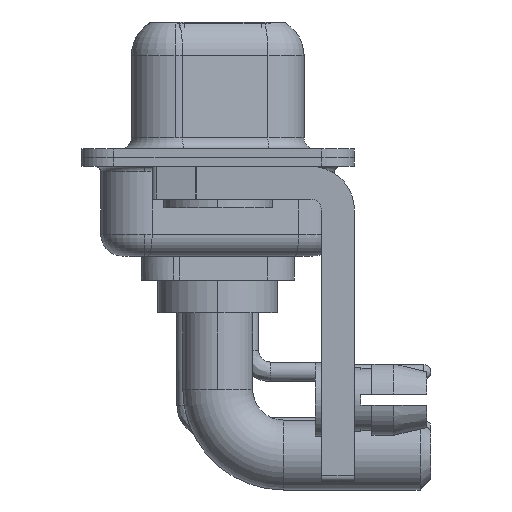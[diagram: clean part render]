
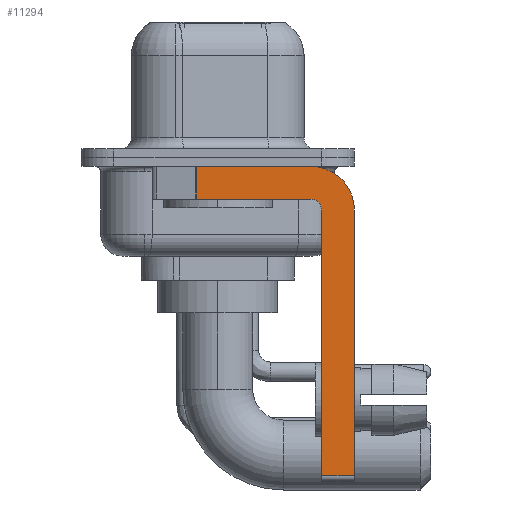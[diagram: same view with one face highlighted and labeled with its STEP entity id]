
A CAD part, left-side view. The second image highlights one B-rep face of the part: STEP entity #11294.
In plain terms, the highlighted planar face has unit normal (-1, 0, 0).
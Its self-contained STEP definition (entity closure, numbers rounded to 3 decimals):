
#166 = VERTEX_POINT ( 'NONE', #17908 ) ;
#473 = VERTEX_POINT ( 'NONE', #15379 ) ;
#1239 = ORIENTED_EDGE ( 'NONE', *, *, #25245, .F. ) ;
#1718 = VECTOR ( 'NONE', #11617, 1000. ) ;
#2003 = CARTESIAN_POINT ( 'NONE',  ( -2.9, -6.25, -2.4 ) ) ;
#2008 = VECTOR ( 'NONE', #10098, 1000. ) ;
#2915 = ORIENTED_EDGE ( 'NONE', *, *, #24611, .F. ) ;
#3667 = PLANE ( 'NONE',  #7235 ) ;
#5119 = CARTESIAN_POINT ( 'NONE',  ( -2.9, 0.978, -1.9 ) ) ;
#5285 = EDGE_CURVE ( 'NONE', #21362, #473, #16288, .T. ) ;
#5353 = CIRCLE ( 'NONE', #13408, 0.5 ) ;
#6689 = CARTESIAN_POINT ( 'NONE',  ( -2.9, -4.25, -2.4 ) ) ;
#6922 = VECTOR ( 'NONE', #20558, 1000. ) ;
#7119 = CARTESIAN_POINT ( 'NONE',  ( -2.9, -4.25, -1.9 ) ) ;
#7217 = VERTEX_POINT ( 'NONE', #15669 ) ;
#7235 = AXIS2_PLACEMENT_3D ( 'NONE', #11904, #17581, #11758 ) ;
#9989 = CARTESIAN_POINT ( 'NONE',  ( -2.9, -4.25, -0.4 ) ) ;
#10098 = DIRECTION ( 'NONE',  ( 0., 0., -1. ) ) ;
#11145 = DIRECTION ( 'NONE',  ( 0., -1., 0. ) ) ;
#11294 = ADVANCED_FACE ( 'NONE', ( #25936 ), #3667, .F. ) ;
#11464 = ORIENTED_EDGE ( 'NONE', *, *, #17153, .T. ) ;
#11617 = DIRECTION ( 'NONE',  ( 0., 0., -1. ) ) ;
#11758 = DIRECTION ( 'NONE',  ( 0., 0., -1. ) ) ;
#11855 = CARTESIAN_POINT ( 'NONE',  ( -2.9, -4.25, -2.4 ) ) ;
#11904 = CARTESIAN_POINT ( 'NONE',  ( -2.9, -4.25, -2.4 ) ) ;
#11932 = VERTEX_POINT ( 'NONE', #5119 ) ;
#12075 = CARTESIAN_POINT ( 'NONE',  ( -2.9, 0.978, -0.4 ) ) ;
#12192 = VECTOR ( 'NONE', #15213, 1000. ) ;
#12328 = DIRECTION ( 'NONE',  ( 0., 0., 1. ) ) ;
#12486 = VECTOR ( 'NONE', #11145, 1000. ) ;
#12495 = CARTESIAN_POINT ( 'NONE',  ( -2.9, 3., -0.4 ) ) ;
#13320 = VERTEX_POINT ( 'NONE', #22904 ) ;
#13378 = VECTOR ( 'NONE', #12328, 1000. ) ;
#13408 = AXIS2_PLACEMENT_3D ( 'NONE', #11855, #19922, #26015 ) ;
#13911 = VERTEX_POINT ( 'NONE', #12075 ) ;
#14338 = ORIENTED_EDGE ( 'NONE', *, *, #22501, .T. ) ;
#14781 = DIRECTION ( 'NONE',  ( 1., 0., 0. ) ) ;
#15213 = DIRECTION ( 'NONE',  ( 0., 1., 0. ) ) ;
#15379 = CARTESIAN_POINT ( 'NONE',  ( -2.9, -4.75, -2.4 ) ) ;
#15669 = CARTESIAN_POINT ( 'NONE',  ( -2.9, -6.25, -14.55 ) ) ;
#16193 = LINE ( 'NONE', #2003, #2008 ) ;
#16288 = LINE ( 'NONE', #20791, #13378 ) ;
#16463 = LINE ( 'NONE', #12495, #6922 ) ;
#17042 = ORIENTED_EDGE ( 'NONE', *, *, #26030, .F. ) ;
#17153 = EDGE_CURVE ( 'NONE', #13911, #11932, #25525, .T. ) ;
#17204 = EDGE_LOOP ( 'NONE', ( #22673, #11464, #17042, #2915, #20929, #14338, #1239, #18710 ) ) ;
#17562 = CARTESIAN_POINT ( 'NONE',  ( -2.9, -4.75, -14.55 ) ) ;
#17581 = DIRECTION ( 'NONE',  ( 1., 0., 0. ) ) ;
#17908 = CARTESIAN_POINT ( 'NONE',  ( -2.9, -6.25, -2.4 ) ) ;
#18710 = ORIENTED_EDGE ( 'NONE', *, *, #20350, .F. ) ;
#19082 = LINE ( 'NONE', #24915, #12486 ) ;
#19922 = DIRECTION ( 'NONE',  ( -1., 0., 0. ) ) ;
#20350 = EDGE_CURVE ( 'NONE', #21792, #166, #22184, .T. ) ;
#20558 = DIRECTION ( 'NONE',  ( 0., -1., 0. ) ) ;
#20674 = EDGE_CURVE ( 'NONE', #13911, #21792, #16463, .T. ) ;
#20791 = CARTESIAN_POINT ( 'NONE',  ( -2.9, -4.75, -14.8 ) ) ;
#20929 = ORIENTED_EDGE ( 'NONE', *, *, #5285, .F. ) ;
#21285 = CARTESIAN_POINT ( 'NONE',  ( -2.9, 0.978, -1.9 ) ) ;
#21362 = VERTEX_POINT ( 'NONE', #17562 ) ;
#21792 = VERTEX_POINT ( 'NONE', #9989 ) ;
#22184 = CIRCLE ( 'NONE', #23871, 2. ) ;
#22501 = EDGE_CURVE ( 'NONE', #21362, #7217, #19082, .T. ) ;
#22673 = ORIENTED_EDGE ( 'NONE', *, *, #20674, .F. ) ;
#22867 = DIRECTION ( 'NONE',  ( 0., 0., -1. ) ) ;
#22904 = CARTESIAN_POINT ( 'NONE',  ( -2.9, -4.25, -1.9 ) ) ;
#23871 = AXIS2_PLACEMENT_3D ( 'NONE', #6689, #14781, #22867 ) ;
#24611 = EDGE_CURVE ( 'NONE', #473, #13320, #5353, .T. ) ;
#24915 = CARTESIAN_POINT ( 'NONE',  ( -2.9, -4.25, -14.55 ) ) ;
#25245 = EDGE_CURVE ( 'NONE', #166, #7217, #16193, .T. ) ;
#25275 = LINE ( 'NONE', #7119, #12192 ) ;
#25525 = LINE ( 'NONE', #21285, #1718 ) ;
#25936 = FACE_OUTER_BOUND ( 'NONE', #17204, .T. ) ;
#26015 = DIRECTION ( 'NONE',  ( 0., 0., 1. ) ) ;
#26030 = EDGE_CURVE ( 'NONE', #13320, #11932, #25275, .T. ) ;
